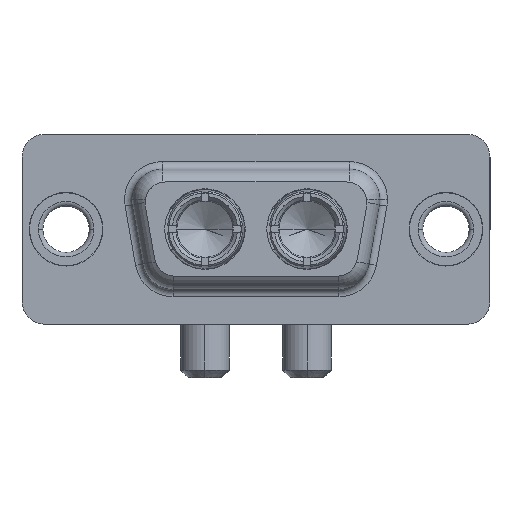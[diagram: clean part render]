
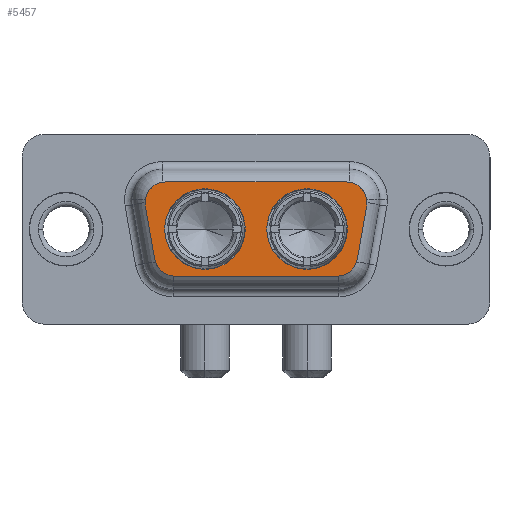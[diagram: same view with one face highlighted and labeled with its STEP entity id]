
A CAD part, top view. The second image highlights one B-rep face of the part: STEP entity #5457.
In plain terms, the highlighted planar face has unit normal (0, 0, 1).
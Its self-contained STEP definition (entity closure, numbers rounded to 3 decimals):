
#25 = AXIS2_PLACEMENT_3D ( 'NONE', #10365, #5528, #8726 ) ;
#31 = DIRECTION ( 'NONE',  ( 0., 0., 1. ) ) ;
#217 = CARTESIAN_POINT ( 'NONE',  ( 6.55, 3.1, 6.2 ) ) ;
#261 = EDGE_LOOP ( 'NONE', ( #7495, #993 ) ) ;
#478 = VERTEX_POINT ( 'NONE', #4944 ) ;
#647 = DIRECTION ( 'NONE',  ( 0., 0., 1. ) ) ;
#722 = VERTEX_POINT ( 'NONE', #10124 ) ;
#756 = FACE_BOUND ( 'NONE', #261, .T. ) ;
#926 = CARTESIAN_POINT ( 'NONE',  ( 6.55, 1.75, 6.2 ) ) ;
#954 = AXIS2_PLACEMENT_3D ( 'NONE', #926, #1034, #5706 ) ;
#983 = DIRECTION ( 'NONE',  ( 1., 0., 0. ) ) ;
#993 = ORIENTED_EDGE ( 'NONE', *, *, #6358, .F. ) ;
#1034 = DIRECTION ( 'NONE',  ( 0., 0., 1. ) ) ;
#1044 = EDGE_CURVE ( 'NONE', #3030, #7943, #4409, .T. ) ;
#1111 = DIRECTION ( 'NONE',  ( 0., 0., 1. ) ) ;
#1116 = CIRCLE ( 'NONE', #954, 1.35 ) ;
#1122 = CARTESIAN_POINT ( 'NONE',  ( 15.86, 0., 6.2 ) ) ;
#1141 = CARTESIAN_POINT ( 'NONE',  ( 9.14, 0., 6.2 ) ) ;
#1158 = CARTESIAN_POINT ( 'NONE',  ( 6.55, 3.1, 6.2 ) ) ;
#1254 = VECTOR ( 'NONE', #5368, 1000. ) ;
#1270 = EDGE_CURVE ( 'NONE', #4833, #8279, #9595, .T. ) ;
#1541 = DIRECTION ( 'NONE',  ( 1., 0., 0. ) ) ;
#1696 = ORIENTED_EDGE ( 'NONE', *, *, #5098, .F. ) ;
#1820 = ORIENTED_EDGE ( 'NONE', *, *, #5390, .F. ) ;
#1895 = CARTESIAN_POINT ( 'NONE',  ( 5.838, -1.984, 6.2 ) ) ;
#1916 = EDGE_CURVE ( 'NONE', #2007, #4833, #9399, .T. ) ;
#1989 = CARTESIAN_POINT ( 'NONE',  ( 6.49, 0., 6.2 ) ) ;
#2007 = VERTEX_POINT ( 'NONE', #8670 ) ;
#2049 = DIRECTION ( 'NONE',  ( 1., 0., 0. ) ) ;
#2070 = EDGE_CURVE ( 'NONE', #722, #5888, #7587, .T. ) ;
#2092 = CIRCLE ( 'NONE', #6802, 1.35 ) ;
#2115 = ORIENTED_EDGE ( 'NONE', *, *, #6612, .T. ) ;
#2172 = CARTESIAN_POINT ( 'NONE',  ( 17.833, -3.1, 6.2 ) ) ;
#2204 = CIRCLE ( 'NONE', #8077, 2.65 ) ;
#2270 = VECTOR ( 'NONE', #5093, 1000. ) ;
#2302 = EDGE_CURVE ( 'NONE', #10178, #478, #9175, .T. ) ;
#2660 = ORIENTED_EDGE ( 'NONE', *, *, #6875, .T. ) ;
#2882 = VECTOR ( 'NONE', #3672, 1000. ) ;
#2892 = ORIENTED_EDGE ( 'NONE', *, *, #1916, .T. ) ;
#2903 = CARTESIAN_POINT ( 'NONE',  ( 17.833, -1.75, 6.2 ) ) ;
#2969 = LINE ( 'NONE', #2172, #1254 ) ;
#3030 = VERTEX_POINT ( 'NONE', #5447 ) ;
#3316 = EDGE_LOOP ( 'NONE', ( #8299, #2660, #2892, #3716, #8102, #9803, #2115, #8334, #3658 ) ) ;
#3658 = ORIENTED_EDGE ( 'NONE', *, *, #6013, .T. ) ;
#3672 = DIRECTION ( 'NONE',  ( -1., 0., 0. ) ) ;
#3716 = ORIENTED_EDGE ( 'NONE', *, *, #1270, .T. ) ;
#3904 = FACE_OUTER_BOUND ( 'NONE', #3316, .T. ) ;
#3991 = DIRECTION ( 'NONE',  ( 0.174, 0.985, 0. ) ) ;
#4068 = CARTESIAN_POINT ( 'NONE',  ( 9.14, 0., 6.2 ) ) ;
#4125 = CARTESIAN_POINT ( 'NONE',  ( 18.51, 0., 6.2 ) ) ;
#4256 = DIRECTION ( 'NONE',  ( -1., 0., 0. ) ) ;
#4382 = CARTESIAN_POINT ( 'NONE',  ( 5.838, -1.984, 6.2 ) ) ;
#4388 = AXIS2_PLACEMENT_3D ( 'NONE', #2903, #7625, #8315 ) ;
#4409 = LINE ( 'NONE', #1158, #2882 ) ;
#4653 = CARTESIAN_POINT ( 'NONE',  ( 19.779, 1.516, 6.2 ) ) ;
#4712 = CARTESIAN_POINT ( 'NONE',  ( 19.779, 1.516, 6.2 ) ) ;
#4739 = CARTESIAN_POINT ( 'NONE',  ( 7.167, -3.1, 6.2 ) ) ;
#4780 = CARTESIAN_POINT ( 'NONE',  ( 5.221, 1.516, 6.2 ) ) ;
#4795 = PLANE ( 'NONE',  #25 ) ;
#4833 = VERTEX_POINT ( 'NONE', #5486 ) ;
#4866 = CARTESIAN_POINT ( 'NONE',  ( 11.79, 0., 6.2 ) ) ;
#4944 = CARTESIAN_POINT ( 'NONE',  ( 13.21, 0., 6.2 ) ) ;
#5093 = DIRECTION ( 'NONE',  ( 0.174, -0.985, 0. ) ) ;
#5098 = EDGE_CURVE ( 'NONE', #8141, #9760, #2204, .T. ) ;
#5134 = AXIS2_PLACEMENT_3D ( 'NONE', #9876, #1111, #2049 ) ;
#5368 = DIRECTION ( 'NONE',  ( 1., 0., 0. ) ) ;
#5390 = EDGE_CURVE ( 'NONE', #9760, #8141, #5722, .T. ) ;
#5447 = CARTESIAN_POINT ( 'NONE',  ( 18.45, 3.1, 6.2 ) ) ;
#5457 = ADVANCED_FACE ( 'NONE', ( #756, #6428, #3904 ), #4795, .F. ) ;
#5486 = CARTESIAN_POINT ( 'NONE',  ( 19.162, -1.984, 6.2 ) ) ;
#5528 = DIRECTION ( 'NONE',  ( 0., 0., -1. ) ) ;
#5605 = AXIS2_PLACEMENT_3D ( 'NONE', #5863, #8379, #6706 ) ;
#5706 = DIRECTION ( 'NONE',  ( 1., 0., 0. ) ) ;
#5722 = CIRCLE ( 'NONE', #6212, 2.65 ) ;
#5784 = VERTEX_POINT ( 'NONE', #4382 ) ;
#5863 = CARTESIAN_POINT ( 'NONE',  ( 18.45, 1.75, 6.2 ) ) ;
#5888 = VERTEX_POINT ( 'NONE', #4780 ) ;
#5889 = DIRECTION ( 'NONE',  ( 0., 0., 1. ) ) ;
#5939 = EDGE_CURVE ( 'NONE', #5784, #10125, #2092, .T. ) ;
#6013 = EDGE_CURVE ( 'NONE', #5888, #5784, #6680, .T. ) ;
#6212 = AXIS2_PLACEMENT_3D ( 'NONE', #4068, #31, #9576 ) ;
#6358 = EDGE_CURVE ( 'NONE', #478, #10178, #7805, .T. ) ;
#6428 = FACE_BOUND ( 'NONE', #7450, .T. ) ;
#6612 = EDGE_CURVE ( 'NONE', #7943, #722, #1116, .T. ) ;
#6680 = LINE ( 'NONE', #1895, #2270 ) ;
#6706 = DIRECTION ( 'NONE',  ( -1., 0., 0. ) ) ;
#6802 = AXIS2_PLACEMENT_3D ( 'NONE', #8886, #9725, #4256 ) ;
#6875 = EDGE_CURVE ( 'NONE', #10125, #2007, #2969, .T. ) ;
#7450 = EDGE_LOOP ( 'NONE', ( #1820, #1696 ) ) ;
#7464 = CIRCLE ( 'NONE', #5605, 1.35 ) ;
#7495 = ORIENTED_EDGE ( 'NONE', *, *, #2302, .F. ) ;
#7567 = DIRECTION ( 'NONE',  ( 1., 0., 0. ) ) ;
#7587 = CIRCLE ( 'NONE', #9597, 1.35 ) ;
#7625 = DIRECTION ( 'NONE',  ( 0., 0., 1. ) ) ;
#7805 = CIRCLE ( 'NONE', #5134, 2.65 ) ;
#7908 = VECTOR ( 'NONE', #3991, 1000. ) ;
#7943 = VERTEX_POINT ( 'NONE', #217 ) ;
#8077 = AXIS2_PLACEMENT_3D ( 'NONE', #1141, #9950, #983 ) ;
#8102 = ORIENTED_EDGE ( 'NONE', *, *, #9951, .T. ) ;
#8141 = VERTEX_POINT ( 'NONE', #1989 ) ;
#8279 = VERTEX_POINT ( 'NONE', #4653 ) ;
#8299 = ORIENTED_EDGE ( 'NONE', *, *, #5939, .T. ) ;
#8315 = DIRECTION ( 'NONE',  ( -1., 0., 0. ) ) ;
#8334 = ORIENTED_EDGE ( 'NONE', *, *, #2070, .T. ) ;
#8379 = DIRECTION ( 'NONE',  ( 0., 0., 1. ) ) ;
#8562 = CARTESIAN_POINT ( 'NONE',  ( 6.55, 1.75, 6.2 ) ) ;
#8670 = CARTESIAN_POINT ( 'NONE',  ( 17.833, -3.1, 6.2 ) ) ;
#8726 = DIRECTION ( 'NONE',  ( -1., 0., 0. ) ) ;
#8886 = CARTESIAN_POINT ( 'NONE',  ( 7.167, -1.75, 6.2 ) ) ;
#9175 = CIRCLE ( 'NONE', #9838, 2.65 ) ;
#9399 = CIRCLE ( 'NONE', #4388, 1.35 ) ;
#9576 = DIRECTION ( 'NONE',  ( 1., 0., 0. ) ) ;
#9595 = LINE ( 'NONE', #4712, #7908 ) ;
#9597 = AXIS2_PLACEMENT_3D ( 'NONE', #8562, #647, #1541 ) ;
#9725 = DIRECTION ( 'NONE',  ( 0., 0., 1. ) ) ;
#9760 = VERTEX_POINT ( 'NONE', #4866 ) ;
#9803 = ORIENTED_EDGE ( 'NONE', *, *, #1044, .T. ) ;
#9838 = AXIS2_PLACEMENT_3D ( 'NONE', #1122, #5889, #7567 ) ;
#9876 = CARTESIAN_POINT ( 'NONE',  ( 15.86, 0., 6.2 ) ) ;
#9950 = DIRECTION ( 'NONE',  ( 0., 0., 1. ) ) ;
#9951 = EDGE_CURVE ( 'NONE', #8279, #3030, #7464, .T. ) ;
#10124 = CARTESIAN_POINT ( 'NONE',  ( 5.2, 1.75, 6.2 ) ) ;
#10125 = VERTEX_POINT ( 'NONE', #4739 ) ;
#10178 = VERTEX_POINT ( 'NONE', #4125 ) ;
#10365 = CARTESIAN_POINT ( 'NONE',  ( 7.167, -1.75, 6.2 ) ) ;
